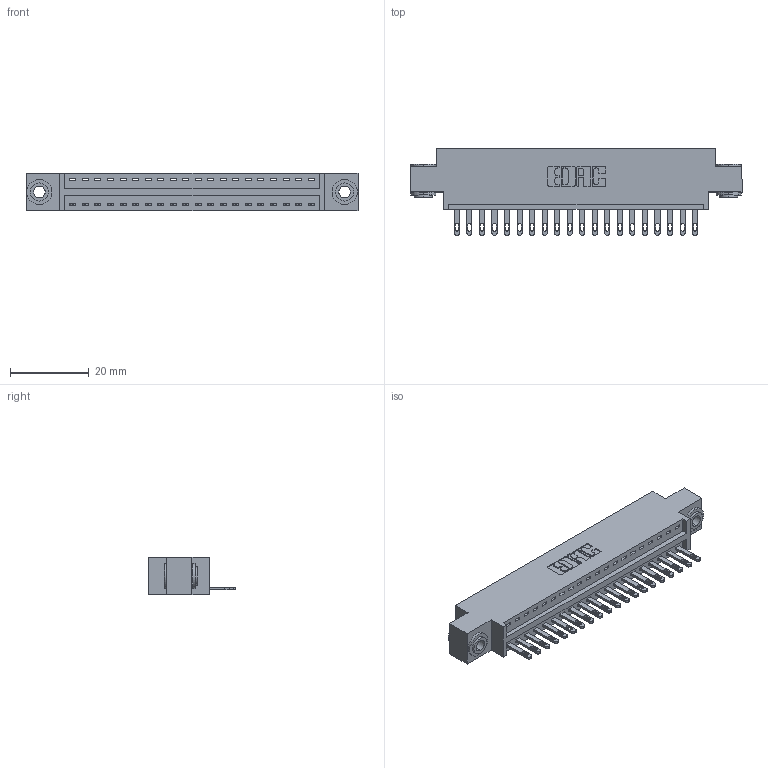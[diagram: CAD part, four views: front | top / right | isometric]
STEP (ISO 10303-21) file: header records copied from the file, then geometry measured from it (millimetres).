
FILE_DESCRIPTION (( 'STEP AP203' ), '1' );
FILE_NAME ('346-020-500-603.STEP', '2018-08-20T10:48:49', ( '' ), ( '' ), 'SwSTEP 2.0', 'SolidWorks 2016', '' );
FILE_SCHEMA (( 'CONFIG_CONTROL_DESIGN' ));
Length unit declared in the file: inch
Products named in the file (4): 346 Part_0.170 Offset - 0.156 Dia-TH; 345-292-001_345-293-100; 345-250-002_345-250-002-102; 346-020-500-603
Assembly tree (23 placements, depth 2):
  346-020-500-603
    346 Part_0.170 Offset - 0.156 Dia-TH
    345-292-001_345-293-100  x20
    345-250-002_345-250-002-102  x2
Bounding box: 84.07 x 21.84 x 9.4 mm (x, y, z)
Volume: 7773.3 mm3; surface area: 9904.4 mm2
Topology: 23 solids, 23 shells, 1244 faces, 3777 edges, 2514 vertices
Faces by surface type: plane 770, cylinder 466, cone 8
Entity records: 16086 total; most frequent: CARTESIAN_POINT 2743, ORIENTED_EDGE 2690, DIRECTION 2479, EDGE_CURVE 1345, VECTOR 1105, LINE 1105, VERTEX_POINT 894, AXIS2_PLACEMENT_3D 687
